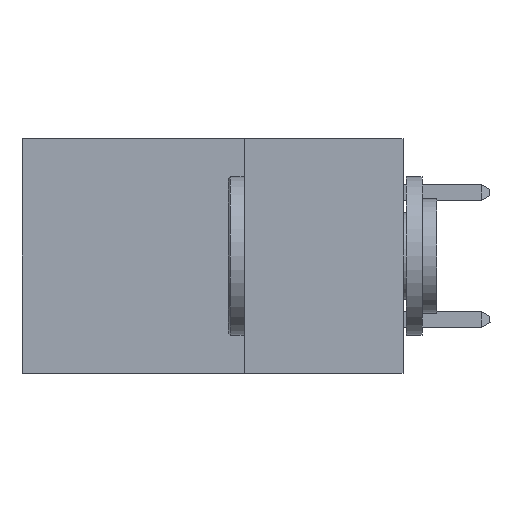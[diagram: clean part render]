
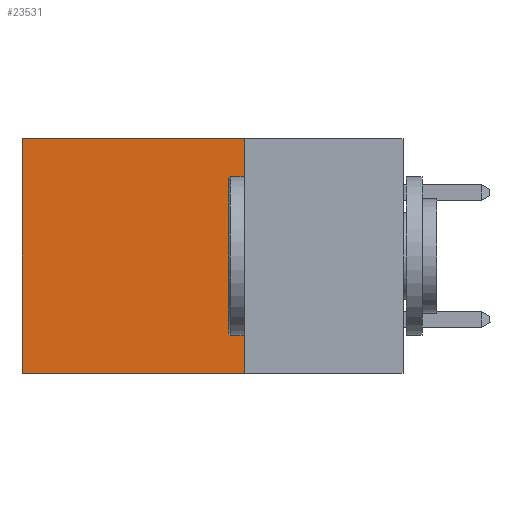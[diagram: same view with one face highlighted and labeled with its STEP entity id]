
A CAD part, left-side view. The second image highlights one B-rep face of the part: STEP entity #23531.
In plain terms, the highlighted planar face has unit normal (-1, 0, 0).
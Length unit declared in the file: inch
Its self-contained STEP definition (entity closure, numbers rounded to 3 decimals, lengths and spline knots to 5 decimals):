
#561 = VECTOR ( 'NONE', #30718, 39.37008 ) ;
#1835 = VERTEX_POINT ( 'NONE', #4646 ) ;
#2294 = DIRECTION ( 'NONE',  ( 0., 0., -1. ) ) ;
#2550 = DIRECTION ( 'NONE',  ( 0., 0., -1. ) ) ;
#2774 = CARTESIAN_POINT ( 'NONE',  ( 0.2875, 0.25, 0. ) ) ;
#4646 = CARTESIAN_POINT ( 'NONE',  ( 0.2875, 0.6, -0.37 ) ) ;
#4840 = DIRECTION ( 'NONE',  ( 0., 0., -1. ) ) ;
#5509 = DIRECTION ( 'NONE',  ( 1., 0., 0. ) ) ;
#5993 = EDGE_CURVE ( 'NONE', #28048, #17841, #14746, .T. ) ;
#11081 = PLANE ( 'NONE',  #33172 ) ;
#12431 = DIRECTION ( 'NONE',  ( 0., 1., 0. ) ) ;
#12941 = CARTESIAN_POINT ( 'NONE',  ( 0.2875, 0.25, 0. ) ) ;
#13152 = EDGE_CURVE ( 'NONE', #28048, #21659, #17999, .T. ) ;
#14746 = LINE ( 'NONE', #12941, #21237 ) ;
#14773 = FACE_OUTER_BOUND ( 'NONE', #24671, .T. ) ;
#17638 = EDGE_CURVE ( 'NONE', #21659, #1835, #33261, .T. ) ;
#17841 = VERTEX_POINT ( 'NONE', #26884 ) ;
#17999 = LINE ( 'NONE', #31343, #19738 ) ;
#19306 = CARTESIAN_POINT ( 'NONE',  ( 0.2875, 0.25, -0.37 ) ) ;
#19738 = VECTOR ( 'NONE', #12431, 39.37008 ) ;
#21237 = VECTOR ( 'NONE', #4840, 39.37008 ) ;
#21572 = ORIENTED_EDGE ( 'NONE', *, *, #34822, .F. ) ;
#21659 = VERTEX_POINT ( 'NONE', #30067 ) ;
#22517 = LINE ( 'NONE', #19306, #561 ) ;
#23531 = ADVANCED_FACE ( 'NONE', ( #14773 ), #11081, .F. ) ;
#24671 = EDGE_LOOP ( 'NONE', ( #26798, #21572, #26044, #27513 ) ) ;
#25962 = VECTOR ( 'NONE', #2294, 39.37008 ) ;
#26044 = ORIENTED_EDGE ( 'NONE', *, *, #5993, .F. ) ;
#26294 = CARTESIAN_POINT ( 'NONE',  ( 0.2875, 0.25, 0. ) ) ;
#26798 = ORIENTED_EDGE ( 'NONE', *, *, #17638, .T. ) ;
#26884 = CARTESIAN_POINT ( 'NONE',  ( 0.2875, 0.25, -0.37 ) ) ;
#27513 = ORIENTED_EDGE ( 'NONE', *, *, #13152, .T. ) ;
#28048 = VERTEX_POINT ( 'NONE', #26294 ) ;
#30067 = CARTESIAN_POINT ( 'NONE',  ( 0.2875, 0.6, 0. ) ) ;
#30193 = CARTESIAN_POINT ( 'NONE',  ( 0.2875, 0.6, 0. ) ) ;
#30718 = DIRECTION ( 'NONE',  ( 0., 1., 0. ) ) ;
#31343 = CARTESIAN_POINT ( 'NONE',  ( 0.2875, 0.25, 0. ) ) ;
#33172 = AXIS2_PLACEMENT_3D ( 'NONE', #2774, #5509, #2550 ) ;
#33261 = LINE ( 'NONE', #30193, #25962 ) ;
#34822 = EDGE_CURVE ( 'NONE', #17841, #1835, #22517, .T. ) ;
